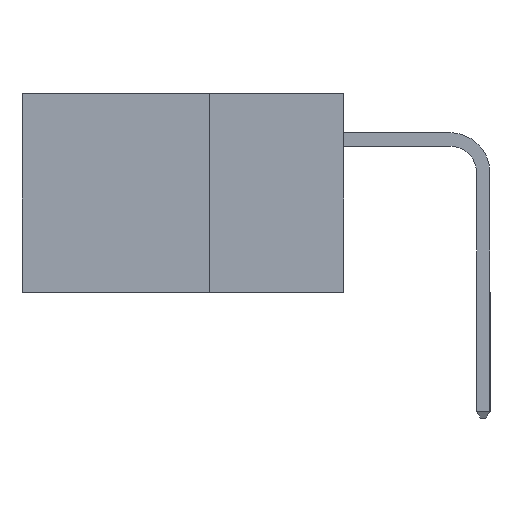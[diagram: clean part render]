
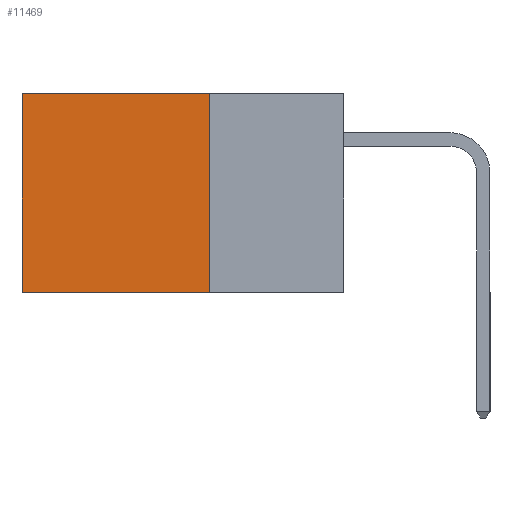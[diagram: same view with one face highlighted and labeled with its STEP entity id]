
A CAD part, left-side view. The second image highlights one B-rep face of the part: STEP entity #11469.
In plain terms, the highlighted planar face has unit normal (-1, 0, 0).
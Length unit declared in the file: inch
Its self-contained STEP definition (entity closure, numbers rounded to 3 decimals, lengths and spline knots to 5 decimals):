
#506 = CARTESIAN_POINT ( 'NONE',  ( 0.298, 0.6, 0. ) ) ;
#2027 = VERTEX_POINT ( 'NONE', #17168 ) ;
#2055 = ORIENTED_EDGE ( 'NONE', *, *, #27945, .F. ) ;
#2409 = DIRECTION ( 'NONE',  ( 1., 0., 0. ) ) ;
#4210 = EDGE_CURVE ( 'NONE', #24266, #25998, #27317, .T. ) ;
#8378 = LINE ( 'NONE', #14360, #20538 ) ;
#10575 = VECTOR ( 'NONE', #13866, 39.37008 ) ;
#11469 = ADVANCED_FACE ( 'NONE', ( #18492 ), #14543, .F. ) ;
#11526 = VECTOR ( 'NONE', #15123, 39.37008 ) ;
#12634 = ORIENTED_EDGE ( 'NONE', *, *, #4210, .T. ) ;
#13354 = VERTEX_POINT ( 'NONE', #18079 ) ;
#13866 = DIRECTION ( 'NONE',  ( 0., 1., 0. ) ) ;
#14360 = CARTESIAN_POINT ( 'NONE',  ( 0.298, 0.25, 0. ) ) ;
#14543 = PLANE ( 'NONE',  #22107 ) ;
#15123 = DIRECTION ( 'NONE',  ( 0., 0., -1. ) ) ;
#15829 = EDGE_LOOP ( 'NONE', ( #26012, #27421, #2055, #12634 ) ) ;
#16813 = DIRECTION ( 'NONE',  ( 0., 0., -1. ) ) ;
#17168 = CARTESIAN_POINT ( 'NONE',  ( 0.298, 0.6, -0.37 ) ) ;
#18079 = CARTESIAN_POINT ( 'NONE',  ( 0.298, 0.25, -0.37 ) ) ;
#18492 = FACE_OUTER_BOUND ( 'NONE', #15829, .T. ) ;
#19354 = CARTESIAN_POINT ( 'NONE',  ( 0.298, 0.6, 0. ) ) ;
#19388 = DIRECTION ( 'NONE',  ( 0., 0., -1. ) ) ;
#20538 = VECTOR ( 'NONE', #16813, 39.37008 ) ;
#20999 = VECTOR ( 'NONE', #27075, 39.37008 ) ;
#21151 = CARTESIAN_POINT ( 'NONE',  ( 0.298, 0.25, -0.37 ) ) ;
#22107 = AXIS2_PLACEMENT_3D ( 'NONE', #31269, #2409, #19388 ) ;
#24226 = LINE ( 'NONE', #21151, #10575 ) ;
#24266 = VERTEX_POINT ( 'NONE', #30779 ) ;
#25098 = LINE ( 'NONE', #506, #11526 ) ;
#25998 = VERTEX_POINT ( 'NONE', #19354 ) ;
#26012 = ORIENTED_EDGE ( 'NONE', *, *, #26703, .T. ) ;
#26703 = EDGE_CURVE ( 'NONE', #25998, #2027, #25098, .T. ) ;
#27075 = DIRECTION ( 'NONE',  ( 0., 1., 0. ) ) ;
#27317 = LINE ( 'NONE', #30916, #20999 ) ;
#27421 = ORIENTED_EDGE ( 'NONE', *, *, #29106, .F. ) ;
#27945 = EDGE_CURVE ( 'NONE', #24266, #13354, #8378, .T. ) ;
#29106 = EDGE_CURVE ( 'NONE', #13354, #2027, #24226, .T. ) ;
#30779 = CARTESIAN_POINT ( 'NONE',  ( 0.298, 0.25, 0. ) ) ;
#30916 = CARTESIAN_POINT ( 'NONE',  ( 0.298, 0.25, 0. ) ) ;
#31269 = CARTESIAN_POINT ( 'NONE',  ( 0.298, 0.25, 0. ) ) ;
